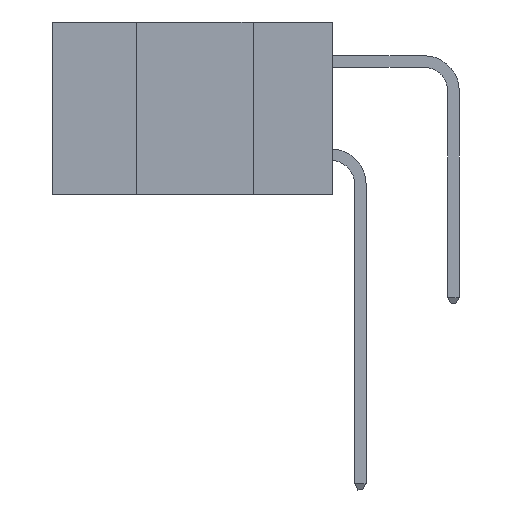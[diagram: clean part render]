
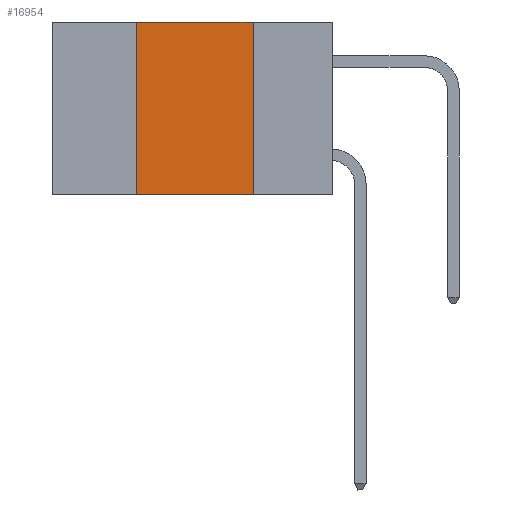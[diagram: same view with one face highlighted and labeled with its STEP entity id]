
A CAD part, left-side view. The second image highlights one B-rep face of the part: STEP entity #16954.
In plain terms, the highlighted planar face has unit normal (-1, 0, 0).
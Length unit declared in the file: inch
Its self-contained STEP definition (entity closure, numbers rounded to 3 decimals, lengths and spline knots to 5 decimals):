
#1366 = VERTEX_POINT ( 'NONE', #10613 ) ;
#1369 = VECTOR ( 'NONE', #19722, 39.37008 ) ;
#1922 = VERTEX_POINT ( 'NONE', #4720 ) ;
#3477 = ORIENTED_EDGE ( 'NONE', *, *, #23045, .F. ) ;
#3556 = CARTESIAN_POINT ( 'NONE',  ( 0., 0.6, -0.37 ) ) ;
#4720 = CARTESIAN_POINT ( 'NONE',  ( 0., 0.17, 0. ) ) ;
#4955 = CARTESIAN_POINT ( 'NONE',  ( 0., 0.17, -0.37 ) ) ;
#5866 = DIRECTION ( 'NONE',  ( 0., -1., 0. ) ) ;
#6781 = LINE ( 'NONE', #7579, #1369 ) ;
#6949 = LINE ( 'NONE', #3556, #21649 ) ;
#7002 = DIRECTION ( 'NONE',  ( 0., 0., -1. ) ) ;
#7091 = CARTESIAN_POINT ( 'NONE',  ( 0., 0.42, 0. ) ) ;
#7450 = DIRECTION ( 'NONE',  ( 1., 0., 0. ) ) ;
#7579 = CARTESIAN_POINT ( 'NONE',  ( 0., 0.42, -0.37 ) ) ;
#8922 = EDGE_LOOP ( 'NONE', ( #13574, #3477, #19499, #14835 ) ) ;
#9447 = VERTEX_POINT ( 'NONE', #7091 ) ;
#10613 = CARTESIAN_POINT ( 'NONE',  ( 0., 0.17, -0.37 ) ) ;
#10974 = EDGE_CURVE ( 'NONE', #18816, #1366, #6949, .T. ) ;
#11304 = CARTESIAN_POINT ( 'NONE',  ( 0., 0.6, 0. ) ) ;
#11984 = VECTOR ( 'NONE', #5866, 39.37008 ) ;
#13574 = ORIENTED_EDGE ( 'NONE', *, *, #25736, .F. ) ;
#14307 = FACE_OUTER_BOUND ( 'NONE', #8922, .T. ) ;
#14328 = CARTESIAN_POINT ( 'NONE',  ( 0., 0.42, -0.37 ) ) ;
#14835 = ORIENTED_EDGE ( 'NONE', *, *, #10974, .T. ) ;
#15304 = VECTOR ( 'NONE', #7002, 39.37008 ) ;
#16377 = EDGE_CURVE ( 'NONE', #18816, #9447, #6781, .T. ) ;
#16697 = LINE ( 'NONE', #17885, #11984 ) ;
#16954 = ADVANCED_FACE ( 'NONE', ( #14307 ), #19445, .F. ) ;
#17496 = AXIS2_PLACEMENT_3D ( 'NONE', #11304, #7450, #21448 ) ;
#17885 = CARTESIAN_POINT ( 'NONE',  ( 0., 0.6, 0. ) ) ;
#18816 = VERTEX_POINT ( 'NONE', #14328 ) ;
#19445 = PLANE ( 'NONE',  #17496 ) ;
#19499 = ORIENTED_EDGE ( 'NONE', *, *, #16377, .F. ) ;
#19619 = DIRECTION ( 'NONE',  ( 0., -1., 0. ) ) ;
#19722 = DIRECTION ( 'NONE',  ( 0., 0., 1. ) ) ;
#20568 = LINE ( 'NONE', #4955, #15304 ) ;
#21448 = DIRECTION ( 'NONE',  ( 0., 0., -1. ) ) ;
#21649 = VECTOR ( 'NONE', #19619, 39.37008 ) ;
#23045 = EDGE_CURVE ( 'NONE', #9447, #1922, #16697, .T. ) ;
#25736 = EDGE_CURVE ( 'NONE', #1922, #1366, #20568, .T. ) ;
